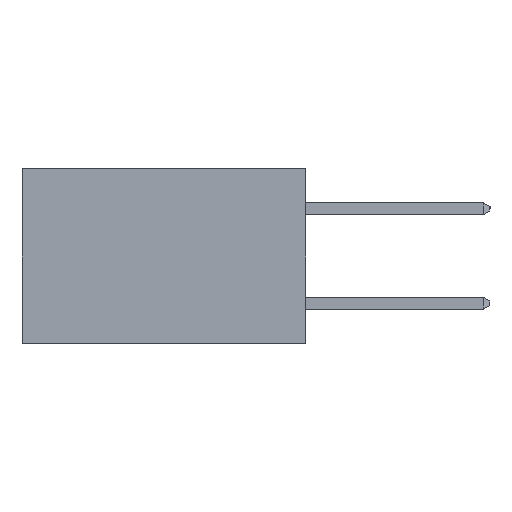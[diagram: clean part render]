
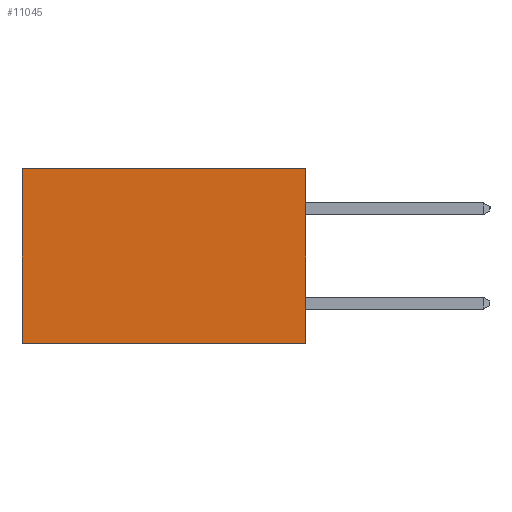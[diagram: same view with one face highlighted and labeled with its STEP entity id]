
A CAD part, left-side view. The second image highlights one B-rep face of the part: STEP entity #11045.
In plain terms, the highlighted planar face has unit normal (-1, 0, 0).
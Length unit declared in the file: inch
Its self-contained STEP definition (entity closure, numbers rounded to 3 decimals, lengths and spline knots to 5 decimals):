
#553 = ORIENTED_EDGE ( 'NONE', *, *, #8707, .T. ) ;
#1484 = PLANE ( 'NONE',  #3004 ) ;
#1578 = CARTESIAN_POINT ( 'NONE',  ( 0.2615, 0., 0. ) ) ;
#1656 = EDGE_CURVE ( 'NONE', #9735, #3887, #14129, .T. ) ;
#1752 = DIRECTION ( 'NONE',  ( 1., 0., 0. ) ) ;
#2314 = LINE ( 'NONE', #4287, #11162 ) ;
#2490 = VERTEX_POINT ( 'NONE', #9769 ) ;
#2848 = FACE_OUTER_BOUND ( 'NONE', #13558, .T. ) ;
#3004 = AXIS2_PLACEMENT_3D ( 'NONE', #11512, #1752, #10680 ) ;
#3184 = CARTESIAN_POINT ( 'NONE',  ( 0.2615, 0.6, -0.37 ) ) ;
#3222 = VECTOR ( 'NONE', #10730, 39.37008 ) ;
#3786 = VERTEX_POINT ( 'NONE', #1578 ) ;
#3887 = VERTEX_POINT ( 'NONE', #3184 ) ;
#4287 = CARTESIAN_POINT ( 'NONE',  ( 0.2615, 0., -0.37 ) ) ;
#4772 = ORIENTED_EDGE ( 'NONE', *, *, #10211, .T. ) ;
#6269 = CARTESIAN_POINT ( 'NONE',  ( 0.2615, 0.6, -0.37 ) ) ;
#6418 = LINE ( 'NONE', #6269, #3222 ) ;
#6814 = ORIENTED_EDGE ( 'NONE', *, *, #10387, .F. ) ;
#8707 = EDGE_CURVE ( 'NONE', #3786, #2490, #11714, .T. ) ;
#8889 = DIRECTION ( 'NONE',  ( 0., 0., -1. ) ) ;
#9370 = CARTESIAN_POINT ( 'NONE',  ( 0.2615, 0., -0.37 ) ) ;
#9735 = VERTEX_POINT ( 'NONE', #14089 ) ;
#9769 = CARTESIAN_POINT ( 'NONE',  ( 0.2615, 0.6, 0. ) ) ;
#10211 = EDGE_CURVE ( 'NONE', #2490, #3887, #6418, .T. ) ;
#10387 = EDGE_CURVE ( 'NONE', #3786, #9735, #2314, .T. ) ;
#10600 = VECTOR ( 'NONE', #12750, 39.37008 ) ;
#10610 = DIRECTION ( 'NONE',  ( 0., 1., 0. ) ) ;
#10680 = DIRECTION ( 'NONE',  ( 0., 0., -1. ) ) ;
#10730 = DIRECTION ( 'NONE',  ( 0., 0., -1. ) ) ;
#11045 = ADVANCED_FACE ( 'NONE', ( #2848 ), #1484, .F. ) ;
#11162 = VECTOR ( 'NONE', #8889, 39.37008 ) ;
#11365 = VECTOR ( 'NONE', #10610, 39.37008 ) ;
#11496 = CARTESIAN_POINT ( 'NONE',  ( 0.2615, 0., 0. ) ) ;
#11512 = CARTESIAN_POINT ( 'NONE',  ( 0.2615, 0., -0.37 ) ) ;
#11714 = LINE ( 'NONE', #11496, #11365 ) ;
#12750 = DIRECTION ( 'NONE',  ( 0., 1., 0. ) ) ;
#12839 = ORIENTED_EDGE ( 'NONE', *, *, #1656, .F. ) ;
#13558 = EDGE_LOOP ( 'NONE', ( #4772, #12839, #6814, #553 ) ) ;
#14089 = CARTESIAN_POINT ( 'NONE',  ( 0.2615, 0., -0.37 ) ) ;
#14129 = LINE ( 'NONE', #9370, #10600 ) ;
